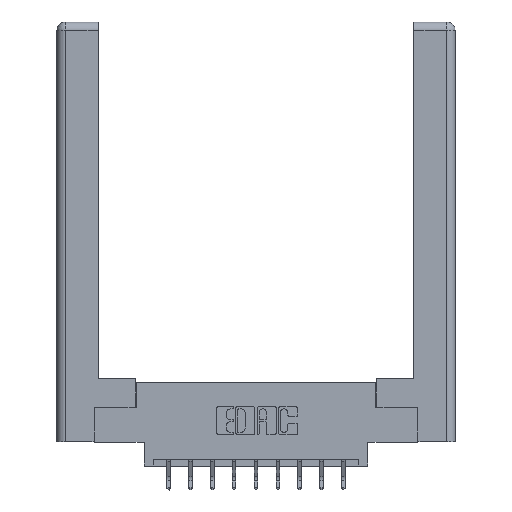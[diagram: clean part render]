
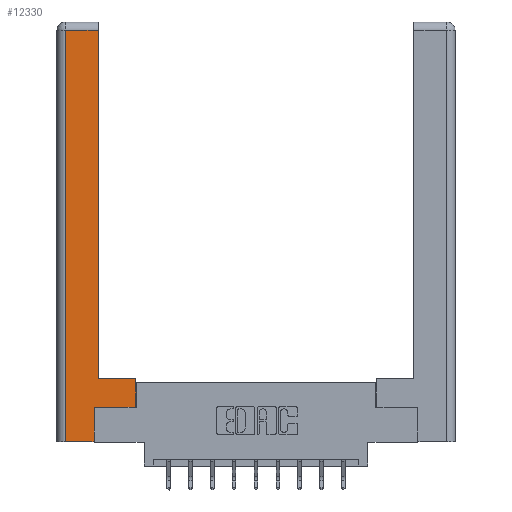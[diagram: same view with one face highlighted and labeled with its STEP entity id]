
A CAD part, top view. The second image highlights one B-rep face of the part: STEP entity #12330.
In plain terms, the highlighted planar face has unit normal (0, 0, 1).
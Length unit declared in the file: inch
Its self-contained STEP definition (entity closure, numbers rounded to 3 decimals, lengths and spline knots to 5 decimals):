
#70 = DIRECTION ( 'NONE',  ( 0., 1., 0. ) ) ;
#233 = DIRECTION ( 'NONE',  ( -1., 0., 0. ) ) ;
#304 = LINE ( 'NONE', #12090, #7718 ) ;
#406 = LINE ( 'NONE', #3899, #13635 ) ;
#502 = EDGE_CURVE ( 'NONE', #14013, #4402, #8204, .T. ) ;
#671 = VERTEX_POINT ( 'NONE', #11790 ) ;
#1092 = EDGE_CURVE ( 'NONE', #6937, #12092, #11134, .T. ) ;
#1105 = VECTOR ( 'NONE', #7872, 39.37008 ) ;
#1260 = FACE_OUTER_BOUND ( 'NONE', #4567, .T. ) ;
#1310 = CARTESIAN_POINT ( 'NONE',  ( 0.565, 0.245, 0. ) ) ;
#1418 = CARTESIAN_POINT ( 'NONE',  ( 0.265, 0., 0. ) ) ;
#1430 = EDGE_CURVE ( 'NONE', #12092, #671, #5796, .T. ) ;
#1799 = VECTOR ( 'NONE', #8935, 39.37008 ) ;
#1969 = EDGE_CURVE ( 'NONE', #11331, #2588, #10223, .T. ) ;
#2091 = CARTESIAN_POINT ( 'NONE',  ( 0.565, 0.45, 0. ) ) ;
#2117 = EDGE_CURVE ( 'NONE', #4402, #11331, #12784, .T. ) ;
#2149 = EDGE_CURVE ( 'NONE', #671, #10858, #6809, .T. ) ;
#2588 = VERTEX_POINT ( 'NONE', #8519 ) ;
#2882 = DIRECTION ( 'NONE',  ( 0., 0., -1. ) ) ;
#3076 = DIRECTION ( 'NONE',  ( -1., 0., 0. ) ) ;
#3422 = CARTESIAN_POINT ( 'NONE',  ( 0.0615, 0., 0. ) ) ;
#3491 = CARTESIAN_POINT ( 'NONE',  ( 0.0615, 0., 0. ) ) ;
#3899 = CARTESIAN_POINT ( 'NONE',  ( 0.265, 0., 0. ) ) ;
#4011 = VECTOR ( 'NONE', #12289, 39.37008 ) ;
#4402 = VERTEX_POINT ( 'NONE', #6206 ) ;
#4434 = CARTESIAN_POINT ( 'NONE',  ( 0.265, 0.245, 0. ) ) ;
#4488 = ORIENTED_EDGE ( 'NONE', *, *, #1092, .T. ) ;
#4567 = EDGE_LOOP ( 'NONE', ( #4488, #10725, #14031, #13737, #10428, #12550, #12892, #7773 ) ) ;
#5024 = DIRECTION ( 'NONE',  ( -1., 0., 0. ) ) ;
#5123 = DIRECTION ( 'NONE',  ( 1., 0., 0. ) ) ;
#5796 = LINE ( 'NONE', #7897, #13022 ) ;
#6206 = CARTESIAN_POINT ( 'NONE',  ( 0.265, 0.245, 0. ) ) ;
#6643 = CARTESIAN_POINT ( 'NONE',  ( 0.295, 3., 0. ) ) ;
#6651 = VECTOR ( 'NONE', #13007, 39.37008 ) ;
#6789 = CARTESIAN_POINT ( 'NONE',  ( 0.295, 2.94, 0. ) ) ;
#6809 = LINE ( 'NONE', #3422, #4011 ) ;
#6937 = VERTEX_POINT ( 'NONE', #10313 ) ;
#7258 = EDGE_CURVE ( 'NONE', #2588, #6937, #304, .T. ) ;
#7718 = VECTOR ( 'NONE', #3076, 39.37008 ) ;
#7773 = ORIENTED_EDGE ( 'NONE', *, *, #7258, .T. ) ;
#7828 = PLANE ( 'NONE',  #12353 ) ;
#7872 = DIRECTION ( 'NONE',  ( 1., 0., 0. ) ) ;
#7876 = CARTESIAN_POINT ( 'NONE',  ( 0., 0., 0. ) ) ;
#7897 = CARTESIAN_POINT ( 'NONE',  ( 0.0615, 2.94, 0. ) ) ;
#8204 = LINE ( 'NONE', #4434, #1799 ) ;
#8519 = CARTESIAN_POINT ( 'NONE',  ( 0.565, 0.45, 0. ) ) ;
#8935 = DIRECTION ( 'NONE',  ( 0., 1., 0. ) ) ;
#9503 = VECTOR ( 'NONE', #70, 39.37008 ) ;
#9881 = EDGE_CURVE ( 'NONE', #10858, #14013, #406, .T. ) ;
#10062 = CARTESIAN_POINT ( 'NONE',  ( 0.565, 0.245, 0. ) ) ;
#10223 = LINE ( 'NONE', #2091, #9503 ) ;
#10313 = CARTESIAN_POINT ( 'NONE',  ( 0.295, 0.45, 0. ) ) ;
#10428 = ORIENTED_EDGE ( 'NONE', *, *, #502, .T. ) ;
#10725 = ORIENTED_EDGE ( 'NONE', *, *, #1430, .T. ) ;
#10858 = VERTEX_POINT ( 'NONE', #3491 ) ;
#11134 = LINE ( 'NONE', #6643, #6651 ) ;
#11331 = VERTEX_POINT ( 'NONE', #10062 ) ;
#11790 = CARTESIAN_POINT ( 'NONE',  ( 0.0615, 2.94, 0. ) ) ;
#12090 = CARTESIAN_POINT ( 'NONE',  ( 0.295, 0.45, 0. ) ) ;
#12092 = VERTEX_POINT ( 'NONE', #6789 ) ;
#12289 = DIRECTION ( 'NONE',  ( 0., -1., 0. ) ) ;
#12330 = ADVANCED_FACE ( 'NONE', ( #1260 ), #7828, .F. ) ;
#12353 = AXIS2_PLACEMENT_3D ( 'NONE', #7876, #2882, #5024 ) ;
#12550 = ORIENTED_EDGE ( 'NONE', *, *, #2117, .T. ) ;
#12784 = LINE ( 'NONE', #1310, #1105 ) ;
#12892 = ORIENTED_EDGE ( 'NONE', *, *, #1969, .T. ) ;
#13007 = DIRECTION ( 'NONE',  ( 0., 1., 0. ) ) ;
#13022 = VECTOR ( 'NONE', #233, 39.37008 ) ;
#13635 = VECTOR ( 'NONE', #5123, 39.37008 ) ;
#13737 = ORIENTED_EDGE ( 'NONE', *, *, #9881, .T. ) ;
#14013 = VERTEX_POINT ( 'NONE', #1418 ) ;
#14031 = ORIENTED_EDGE ( 'NONE', *, *, #2149, .T. ) ;
